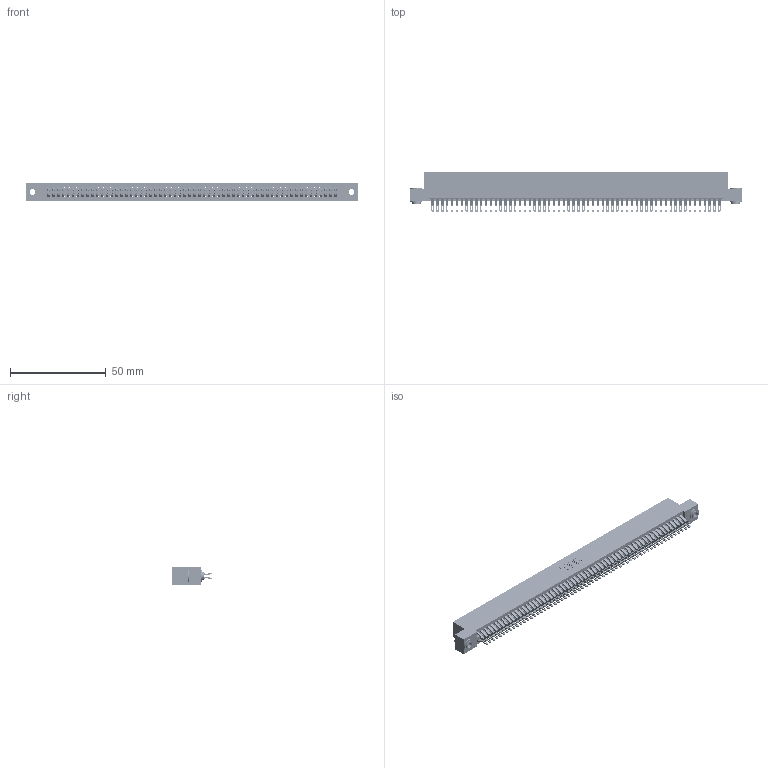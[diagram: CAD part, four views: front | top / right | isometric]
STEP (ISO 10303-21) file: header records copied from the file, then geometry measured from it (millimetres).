
FILE_DESCRIPTION (( 'STEP AP203' ), '1' );
FILE_NAME ('845-120-555-203.STEP', '2018-11-21T05:10:56', ( '' ), ( '' ), 'SwSTEP 2.0', 'SolidWorks 2016', '' );
FILE_SCHEMA (( 'CONFIG_CONTROL_DESIGN' ));
Length unit declared in the file: inch
Products named in the file (4): 845 Part_Flush Mounting Lugs - 0.156 Dia-TH; 345-292-001_555 Tail; 345-250-002_345-250-002-102; 845-120-555-203
Assembly tree (123 placements, depth 2):
  845-120-555-203
    845 Part_Flush Mounting Lugs - 0.156 Dia-TH
    345-292-001_555 Tail  x120
    345-250-002_345-250-002-102  x2
Bounding box: 173.61 x 21.13 x 9.4 mm (x, y, z)
Volume: 17399.1 mm3; surface area: 27482.9 mm2
Topology: 123 solids, 123 shells, 6884 faces, 21657 edges, 14434 vertices
Faces by surface type: plane 3810, cylinder 3066, cone 8
Entity records: 45630 total; most frequent: CARTESIAN_POINT 7641, ORIENTED_EDGE 7538, DIRECTION 6715, EDGE_CURVE 3769, LINE 3353, VECTOR 3353, VERTEX_POINT 2510, AXIS2_PLACEMENT_3D 1681
